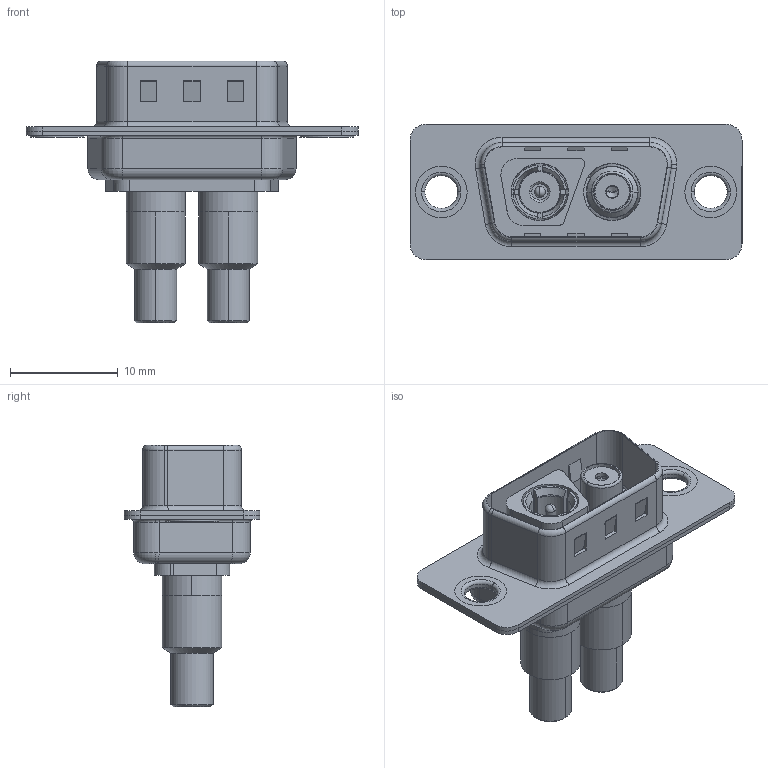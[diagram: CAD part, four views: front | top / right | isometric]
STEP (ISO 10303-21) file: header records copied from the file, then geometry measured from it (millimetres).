
FILE_DESCRIPTION (( 'STEP AP203' ), '1' );
FILE_NAME ('627-2WK2222-5T1.STEP', '2019-05-24T00:32:11', ( '' ), ( '' ), 'SwSTEP 2.0', 'SolidWorks 2016', '' );
FILE_SCHEMA (( 'CONFIG_CONTROL_DESIGN' ));
Length unit declared in the file: millimetre
Products named in the file (16): Co-Ax Jack_Solder Cup Tail; 627Combo Shell Front_09 Contacts; Insulator Socket; 627Combo Thru Hole Rivet; Insulator Socket 2; Co-Ax Plug_Solder Cup Tail; Socket_Solder Cup; Insulator Pin_Solder Cup Tail; Co-Ax Jack Assy_SC; Pin_Solder Cup; 627-2WK2222-5T1; Locking Collar; Solder Cover; 627Combo Housing_2WK2; Co-Ax Plug Assy_SC; 627Combo Shell Rear_09 Contacts
Assembly tree (18 placements, depth 3):
  627-2WK2222-5T1
    627Combo Housing_2WK2
    627Combo Shell Rear_09 Contacts
    627Combo Shell Front_09 Contacts
    627Combo Thru Hole Rivet  x2
    Co-Ax Plug Assy_SC
      Co-Ax Plug_Solder Cup Tail
      Insulator Pin_Solder Cup Tail
      Pin_Solder Cup
      Locking Collar
      Solder Cover
    Co-Ax Jack Assy_SC
      Co-Ax Jack_Solder Cup Tail
      Insulator Socket
      Insulator Socket 2
      Locking Collar
      Socket_Solder Cup
      Solder Cover
Bounding box: 30.8 x 12.6 x 24.3 mm (x, y, z)
Volume: 1600.4 mm3; surface area: 5283.2 mm2
Topology: 16 solids, 16 shells, 564 faces, 1336 edges, 826 vertices
Faces by surface type: cylinder 244, plane 202, torus 66, cone 46, bspline 4, sphere 2
Entity records: 17140 total; most frequent: CARTESIAN_POINT 2863, DIRECTION 2839, ORIENTED_EDGE 2462, EDGE_CURVE 1231, AXIS2_PLACEMENT_3D 1115, VERTEX_POINT 770, VECTOR 609, LINE 609
